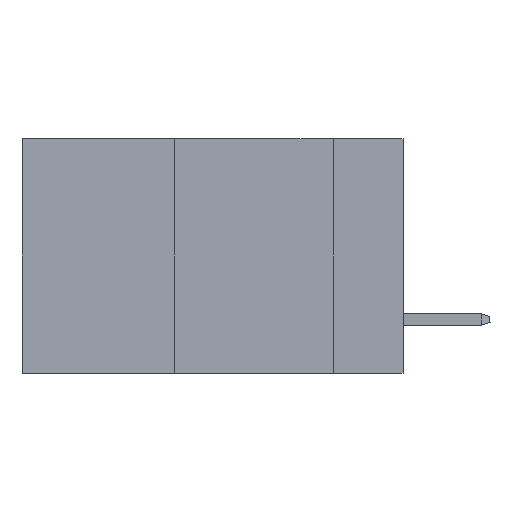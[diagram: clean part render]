
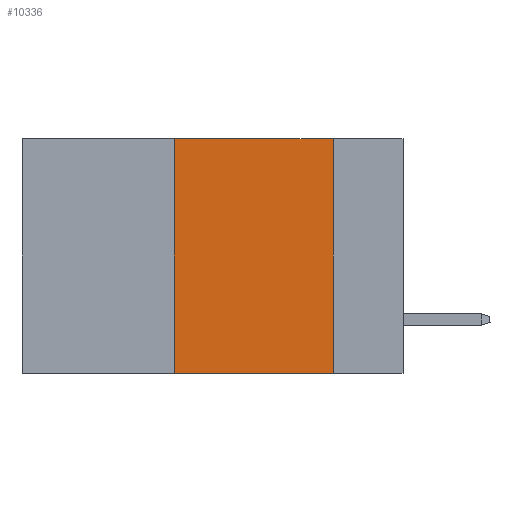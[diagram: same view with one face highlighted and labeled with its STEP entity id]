
A CAD part, left-side view. The second image highlights one B-rep face of the part: STEP entity #10336.
In plain terms, the highlighted planar face has unit normal (-1, 0, 0).
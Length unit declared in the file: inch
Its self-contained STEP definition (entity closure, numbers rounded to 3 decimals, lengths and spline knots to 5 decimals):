
#337 = DIRECTION ( 'NONE',  ( 0., -1., 0. ) ) ;
#1087 = LINE ( 'NONE', #2414, #16422 ) ;
#1663 = EDGE_CURVE ( 'NONE', #13153, #9889, #2318, .T. ) ;
#1842 = CARTESIAN_POINT ( 'NONE',  ( 0., 0.36, 0. ) ) ;
#1955 = CARTESIAN_POINT ( 'NONE',  ( 0., 0.6, -0.37 ) ) ;
#2318 = LINE ( 'NONE', #12518, #11861 ) ;
#2414 = CARTESIAN_POINT ( 'NONE',  ( 0., 0.11, 0. ) ) ;
#2695 = DIRECTION ( 'NONE',  ( 1., 0., 0. ) ) ;
#4146 = PLANE ( 'NONE',  #4470 ) ;
#4468 = FACE_OUTER_BOUND ( 'NONE', #4481, .T. ) ;
#4470 = AXIS2_PLACEMENT_3D ( 'NONE', #17674, #2695, #9244 ) ;
#4481 = EDGE_LOOP ( 'NONE', ( #8529, #9441, #21677, #20534 ) ) ;
#5565 = CARTESIAN_POINT ( 'NONE',  ( 0., 0.11, 0. ) ) ;
#6121 = VECTOR ( 'NONE', #7267, 39.37008 ) ;
#6145 = CARTESIAN_POINT ( 'NONE',  ( 0., 0.11, -0.37 ) ) ;
#7267 = DIRECTION ( 'NONE',  ( 0., 0., 1. ) ) ;
#8529 = ORIENTED_EDGE ( 'NONE', *, *, #15182, .F. ) ;
#9244 = DIRECTION ( 'NONE',  ( 0., 0., -1. ) ) ;
#9441 = ORIENTED_EDGE ( 'NONE', *, *, #1663, .F. ) ;
#9889 = VERTEX_POINT ( 'NONE', #5565 ) ;
#10336 = ADVANCED_FACE ( 'NONE', ( #4468 ), #4146, .F. ) ;
#11861 = VECTOR ( 'NONE', #337, 39.37008 ) ;
#12194 = CARTESIAN_POINT ( 'NONE',  ( 0., 0.36, -0.37 ) ) ;
#12518 = CARTESIAN_POINT ( 'NONE',  ( 0., 0.6, 0. ) ) ;
#12735 = DIRECTION ( 'NONE',  ( 0., 0., -1. ) ) ;
#13153 = VERTEX_POINT ( 'NONE', #1842 ) ;
#14302 = VECTOR ( 'NONE', #17258, 39.37008 ) ;
#14478 = CARTESIAN_POINT ( 'NONE',  ( 0., 0.36, 0. ) ) ;
#15182 = EDGE_CURVE ( 'NONE', #9889, #15797, #1087, .T. ) ;
#15415 = EDGE_CURVE ( 'NONE', #18732, #15797, #18710, .T. ) ;
#15595 = EDGE_CURVE ( 'NONE', #18732, #13153, #16123, .T. ) ;
#15797 = VERTEX_POINT ( 'NONE', #6145 ) ;
#16123 = LINE ( 'NONE', #14478, #6121 ) ;
#16422 = VECTOR ( 'NONE', #12735, 39.37008 ) ;
#17258 = DIRECTION ( 'NONE',  ( 0., -1., 0. ) ) ;
#17674 = CARTESIAN_POINT ( 'NONE',  ( 0., 0.6, 0. ) ) ;
#18710 = LINE ( 'NONE', #1955, #14302 ) ;
#18732 = VERTEX_POINT ( 'NONE', #12194 ) ;
#20534 = ORIENTED_EDGE ( 'NONE', *, *, #15415, .T. ) ;
#21677 = ORIENTED_EDGE ( 'NONE', *, *, #15595, .F. ) ;
